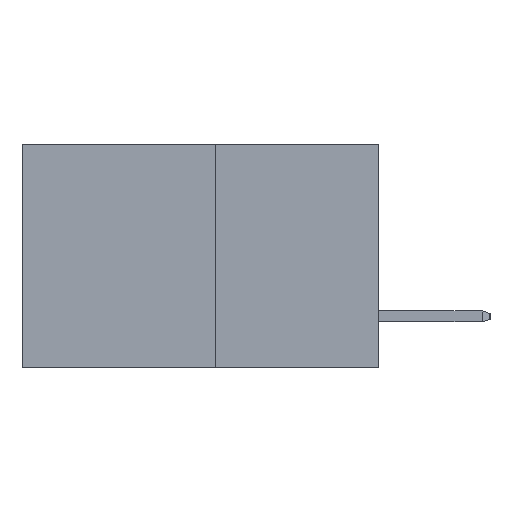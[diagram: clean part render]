
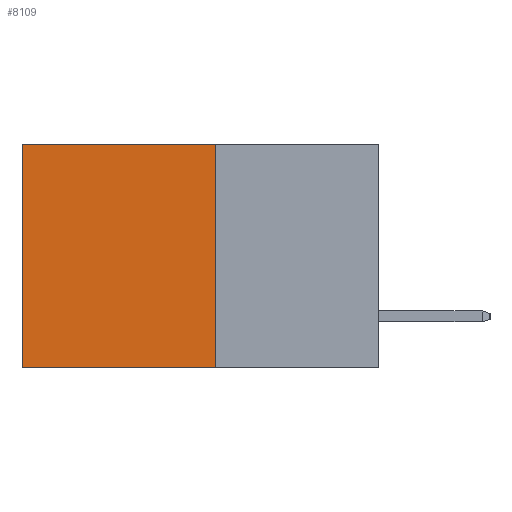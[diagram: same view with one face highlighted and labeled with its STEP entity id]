
A CAD part, left-side view. The second image highlights one B-rep face of the part: STEP entity #8109.
In plain terms, the highlighted planar face has unit normal (-1, 0, 0).
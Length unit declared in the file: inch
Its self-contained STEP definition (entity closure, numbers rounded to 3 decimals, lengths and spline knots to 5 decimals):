
#241 = CARTESIAN_POINT ( 'NONE',  ( 0.277, 0.27, -0.37 ) ) ;
#271 = CARTESIAN_POINT ( 'NONE',  ( 0.277, 0.27, 0. ) ) ;
#446 = DIRECTION ( 'NONE',  ( 1., 0., 0. ) ) ;
#467 = CARTESIAN_POINT ( 'NONE',  ( 0.277, 0.59, 0. ) ) ;
#1344 = LINE ( 'NONE', #9609, #7464 ) ;
#1975 = CARTESIAN_POINT ( 'NONE',  ( 0.277, 0.27, -0.37 ) ) ;
#2247 = AXIS2_PLACEMENT_3D ( 'NONE', #4551, #446, #6088 ) ;
#3205 = VERTEX_POINT ( 'NONE', #5241 ) ;
#3953 = VERTEX_POINT ( 'NONE', #467 ) ;
#4068 = VECTOR ( 'NONE', #7490, 39.37008 ) ;
#4281 = CARTESIAN_POINT ( 'NONE',  ( 0.277, 0.59, -0.37 ) ) ;
#4384 = EDGE_CURVE ( 'NONE', #3205, #3953, #7137, .T. ) ;
#4449 = DIRECTION ( 'NONE',  ( 0., 1., 0. ) ) ;
#4551 = CARTESIAN_POINT ( 'NONE',  ( 0.277, 0.27, -0.37 ) ) ;
#4754 = EDGE_LOOP ( 'NONE', ( #6320, #10108, #8127, #9888 ) ) ;
#5001 = VERTEX_POINT ( 'NONE', #4281 ) ;
#5090 = VECTOR ( 'NONE', #10207, 39.37008 ) ;
#5241 = CARTESIAN_POINT ( 'NONE',  ( 0.277, 0.27, 0. ) ) ;
#5314 = CARTESIAN_POINT ( 'NONE',  ( 0.277, 0.59, -0.37 ) ) ;
#5363 = DIRECTION ( 'NONE',  ( 0., 0., -1. ) ) ;
#5445 = EDGE_CURVE ( 'NONE', #3205, #6031, #9941, .T. ) ;
#5552 = EDGE_CURVE ( 'NONE', #6031, #5001, #1344, .T. ) ;
#6031 = VERTEX_POINT ( 'NONE', #241 ) ;
#6088 = DIRECTION ( 'NONE',  ( 0., 0., -1. ) ) ;
#6104 = LINE ( 'NONE', #5314, #10132 ) ;
#6320 = ORIENTED_EDGE ( 'NONE', *, *, #6788, .T. ) ;
#6788 = EDGE_CURVE ( 'NONE', #3953, #5001, #6104, .T. ) ;
#7137 = LINE ( 'NONE', #271, #5090 ) ;
#7464 = VECTOR ( 'NONE', #4449, 39.37008 ) ;
#7490 = DIRECTION ( 'NONE',  ( 0., 0., -1. ) ) ;
#8109 = ADVANCED_FACE ( 'NONE', ( #9452 ), #9153, .F. ) ;
#8127 = ORIENTED_EDGE ( 'NONE', *, *, #5445, .F. ) ;
#9153 = PLANE ( 'NONE',  #2247 ) ;
#9452 = FACE_OUTER_BOUND ( 'NONE', #4754, .T. ) ;
#9609 = CARTESIAN_POINT ( 'NONE',  ( 0.277, 0.27, -0.37 ) ) ;
#9888 = ORIENTED_EDGE ( 'NONE', *, *, #4384, .T. ) ;
#9941 = LINE ( 'NONE', #1975, #4068 ) ;
#10108 = ORIENTED_EDGE ( 'NONE', *, *, #5552, .F. ) ;
#10132 = VECTOR ( 'NONE', #5363, 39.37008 ) ;
#10207 = DIRECTION ( 'NONE',  ( 0., 1., 0. ) ) ;
